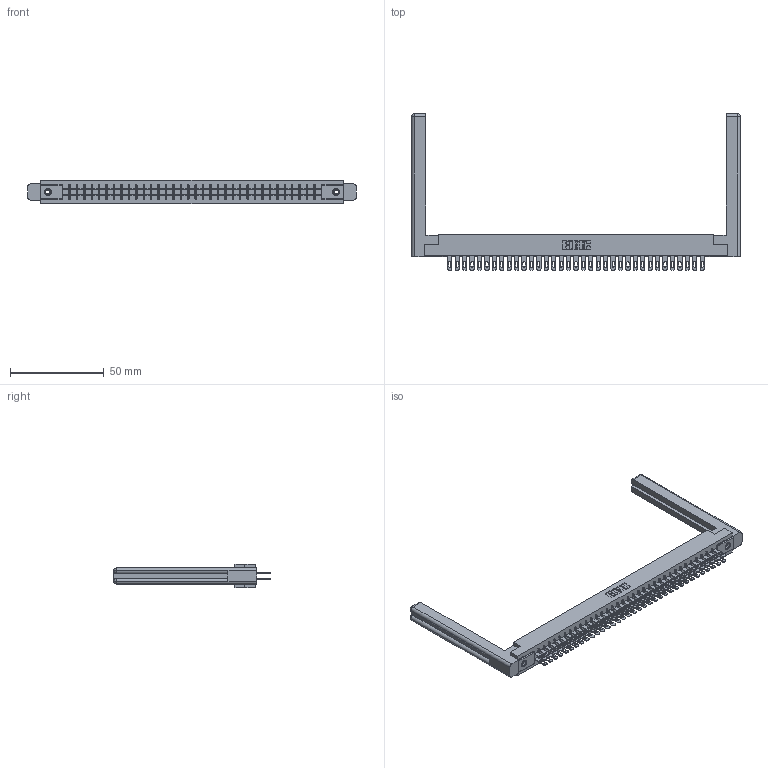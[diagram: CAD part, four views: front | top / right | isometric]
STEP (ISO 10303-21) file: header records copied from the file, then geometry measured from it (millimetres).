
FILE_DESCRIPTION (( 'STEP AP203' ), '1' );
FILE_NAME ('305-070-500-258.STEP', '2019-09-10T04:56:00', ( '' ), ( '' ), 'SwSTEP 2.0', 'SolidWorks 2016', '' );
FILE_SCHEMA (( 'CONFIG_CONTROL_DESIGN' ));
Length unit declared in the file: inch
Products named in the file (5): 305-070-500-258; 307-220-058; 345-250-001_345-250-001-102; 305 Part_.156 Dia; 305-290-001_500
Assembly tree (75 placements, depth 2):
  305-070-500-258
    305 Part_.156 Dia
    305-290-001_500  x70
    345-250-001_345-250-001-102  x2
    307-220-058  x2
Bounding box: 175.31 x 83.49 x 12.7 mm (x, y, z)
Volume: 25614.8 mm3; surface area: 29561.5 mm2
Topology: 75 solids, 75 shells, 3758 faces, 10715 edges, 6942 vertices
Faces by surface type: plane 2112, cylinder 1482, sphere 140, cone 12, torus 12
Entity records: 41403 total; most frequent: CARTESIAN_POINT 6866, ORIENTED_EDGE 6756, DIRECTION 6612, EDGE_CURVE 3378, LINE 2712, VECTOR 2712, VERTEX_POINT 2150, AXIS2_PLACEMENT_3D 1950
